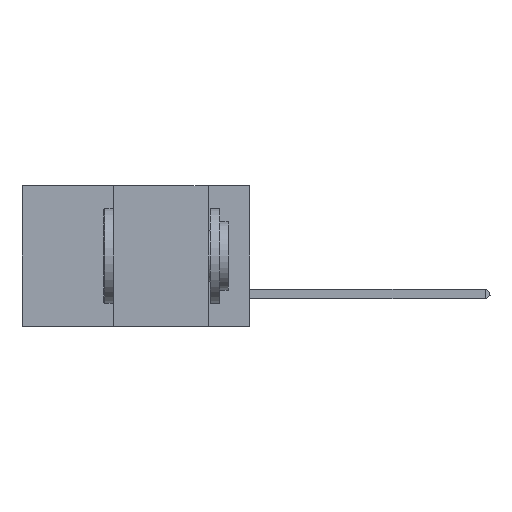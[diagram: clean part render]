
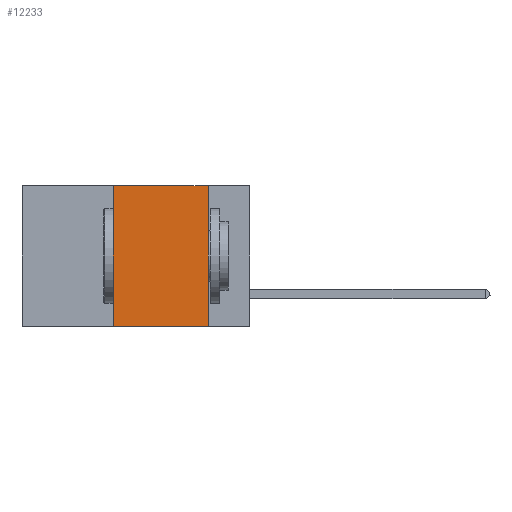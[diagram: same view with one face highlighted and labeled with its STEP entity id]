
A CAD part, left-side view. The second image highlights one B-rep face of the part: STEP entity #12233.
In plain terms, the highlighted planar face has unit normal (-1, 0, 0).
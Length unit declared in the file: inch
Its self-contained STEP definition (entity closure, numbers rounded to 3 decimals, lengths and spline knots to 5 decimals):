
#604 = EDGE_CURVE ( 'NONE', #16159, #2280, #8775, .T. ) ;
#2280 = VERTEX_POINT ( 'NONE', #30458 ) ;
#2600 = DIRECTION ( 'NONE',  ( 0., -1., 0. ) ) ;
#6703 = DIRECTION ( 'NONE',  ( 0., 0., 1. ) ) ;
#6747 = VECTOR ( 'NONE', #9017, 39.37008 ) ;
#8295 = FACE_OUTER_BOUND ( 'NONE', #30035, .T. ) ;
#8775 = LINE ( 'NONE', #12441, #6747 ) ;
#9017 = DIRECTION ( 'NONE',  ( 0., -1., 0. ) ) ;
#9325 = ORIENTED_EDGE ( 'NONE', *, *, #31625, .F. ) ;
#9389 = LINE ( 'NONE', #29882, #24464 ) ;
#12233 = ADVANCED_FACE ( 'NONE', ( #8295 ), #27598, .F. ) ;
#12441 = CARTESIAN_POINT ( 'NONE',  ( 0., 0.6, -0.37 ) ) ;
#12519 = DIRECTION ( 'NONE',  ( 0., 0., -1. ) ) ;
#12884 = VECTOR ( 'NONE', #12519, 39.37008 ) ;
#13708 = LINE ( 'NONE', #15143, #12884 ) ;
#14748 = CARTESIAN_POINT ( 'NONE',  ( 0., 0.36, -0.37 ) ) ;
#14861 = AXIS2_PLACEMENT_3D ( 'NONE', #32505, #30199, #29759 ) ;
#15143 = CARTESIAN_POINT ( 'NONE',  ( 0., 0.11, 0. ) ) ;
#16038 = VERTEX_POINT ( 'NONE', #21812 ) ;
#16159 = VERTEX_POINT ( 'NONE', #14748 ) ;
#18542 = EDGE_CURVE ( 'NONE', #16038, #23362, #22620, .T. ) ;
#20159 = ORIENTED_EDGE ( 'NONE', *, *, #18542, .F. ) ;
#20486 = ORIENTED_EDGE ( 'NONE', *, *, #29548, .F. ) ;
#21812 = CARTESIAN_POINT ( 'NONE',  ( 0., 0.36, 0. ) ) ;
#21819 = VECTOR ( 'NONE', #2600, 39.37008 ) ;
#22620 = LINE ( 'NONE', #23785, #21819 ) ;
#23362 = VERTEX_POINT ( 'NONE', #31426 ) ;
#23785 = CARTESIAN_POINT ( 'NONE',  ( 0., 0.6, 0. ) ) ;
#24464 = VECTOR ( 'NONE', #6703, 39.37008 ) ;
#27598 = PLANE ( 'NONE',  #14861 ) ;
#29548 = EDGE_CURVE ( 'NONE', #16159, #16038, #9389, .T. ) ;
#29759 = DIRECTION ( 'NONE',  ( 0., 0., -1. ) ) ;
#29882 = CARTESIAN_POINT ( 'NONE',  ( 0., 0.36, 0. ) ) ;
#30035 = EDGE_LOOP ( 'NONE', ( #9325, #20159, #20486, #33600 ) ) ;
#30199 = DIRECTION ( 'NONE',  ( 1., 0., 0. ) ) ;
#30458 = CARTESIAN_POINT ( 'NONE',  ( 0., 0.11, -0.37 ) ) ;
#31426 = CARTESIAN_POINT ( 'NONE',  ( 0., 0.11, 0. ) ) ;
#31625 = EDGE_CURVE ( 'NONE', #23362, #2280, #13708, .T. ) ;
#32505 = CARTESIAN_POINT ( 'NONE',  ( 0., 0.6, 0. ) ) ;
#33600 = ORIENTED_EDGE ( 'NONE', *, *, #604, .T. ) ;
